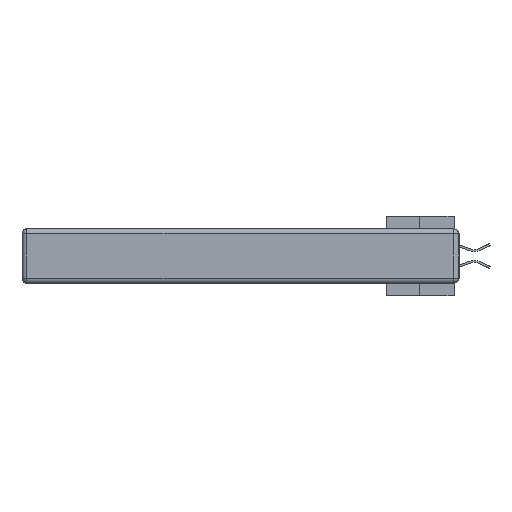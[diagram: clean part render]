
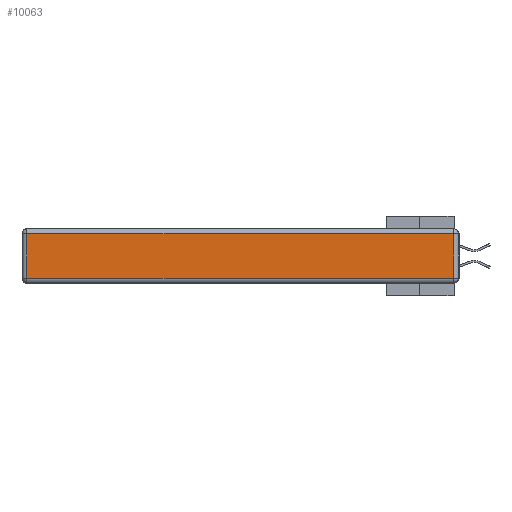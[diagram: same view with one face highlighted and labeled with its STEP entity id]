
A CAD part, left-side view. The second image highlights one B-rep face of the part: STEP entity #10063.
In plain terms, the highlighted planar face has unit normal (-1, 0, 0).
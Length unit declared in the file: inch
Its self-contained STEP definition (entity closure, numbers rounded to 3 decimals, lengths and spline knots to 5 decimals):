
#592 = EDGE_CURVE ( 'NONE', #22662, #6159, #13989, .T. ) ;
#701 = CARTESIAN_POINT ( 'NONE',  ( 0., 2.72, -0.313 ) ) ;
#1378 = LINE ( 'NONE', #16349, #6255 ) ;
#2097 = DIRECTION ( 'NONE',  ( 0., 0., 1. ) ) ;
#2594 = ORIENTED_EDGE ( 'NONE', *, *, #10067, .T. ) ;
#2733 = ORIENTED_EDGE ( 'NONE', *, *, #14937, .T. ) ;
#3500 = AXIS2_PLACEMENT_3D ( 'NONE', #22346, #30597, #22125 ) ;
#6138 = CARTESIAN_POINT ( 'NONE',  ( 0., 2.72, -0.343 ) ) ;
#6159 = VERTEX_POINT ( 'NONE', #15473 ) ;
#6255 = VECTOR ( 'NONE', #2097, 39.37008 ) ;
#7931 = VERTEX_POINT ( 'NONE', #701 ) ;
#8531 = VERTEX_POINT ( 'NONE', #11257 ) ;
#10063 = ADVANCED_FACE ( 'NONE', ( #35705 ), #16454, .T. ) ;
#10067 = EDGE_CURVE ( 'NONE', #8531, #22662, #1378, .T. ) ;
#11257 = CARTESIAN_POINT ( 'NONE',  ( 0., 0.03, -0.313 ) ) ;
#12141 = EDGE_CURVE ( 'NONE', #7931, #8531, #12293, .T. ) ;
#12293 = LINE ( 'NONE', #18080, #36449 ) ;
#13989 = LINE ( 'NONE', #28579, #30983 ) ;
#14937 = EDGE_CURVE ( 'NONE', #6159, #7931, #35889, .T. ) ;
#15473 = CARTESIAN_POINT ( 'NONE',  ( 0., 2.72, -0.03 ) ) ;
#16349 = CARTESIAN_POINT ( 'NONE',  ( 0., 0.03, -0.343 ) ) ;
#16454 = PLANE ( 'NONE',  #3500 ) ;
#17323 = DIRECTION ( 'NONE',  ( 0., 1., 0. ) ) ;
#18080 = CARTESIAN_POINT ( 'NONE',  ( 0., 0., -0.313 ) ) ;
#21820 = DIRECTION ( 'NONE',  ( 0., -1., 0. ) ) ;
#22020 = VECTOR ( 'NONE', #31805, 39.37008 ) ;
#22125 = DIRECTION ( 'NONE',  ( 0., 0., 1. ) ) ;
#22346 = CARTESIAN_POINT ( 'NONE',  ( 0., 0., -0.343 ) ) ;
#22662 = VERTEX_POINT ( 'NONE', #29076 ) ;
#23473 = ORIENTED_EDGE ( 'NONE', *, *, #12141, .T. ) ;
#25773 = EDGE_LOOP ( 'NONE', ( #23473, #2594, #34292, #2733 ) ) ;
#28579 = CARTESIAN_POINT ( 'NONE',  ( 0., 2.75, -0.03 ) ) ;
#29076 = CARTESIAN_POINT ( 'NONE',  ( 0., 0.03, -0.03 ) ) ;
#30597 = DIRECTION ( 'NONE',  ( -1., 0., 0. ) ) ;
#30983 = VECTOR ( 'NONE', #17323, 39.37008 ) ;
#31805 = DIRECTION ( 'NONE',  ( 0., 0., -1. ) ) ;
#34292 = ORIENTED_EDGE ( 'NONE', *, *, #592, .T. ) ;
#35705 = FACE_OUTER_BOUND ( 'NONE', #25773, .T. ) ;
#35889 = LINE ( 'NONE', #6138, #22020 ) ;
#36449 = VECTOR ( 'NONE', #21820, 39.37008 ) ;
